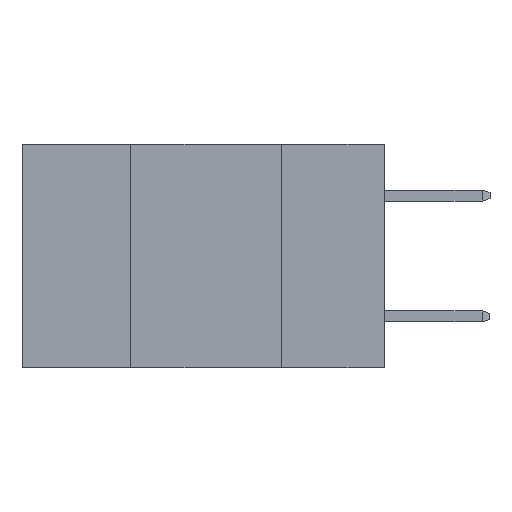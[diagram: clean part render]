
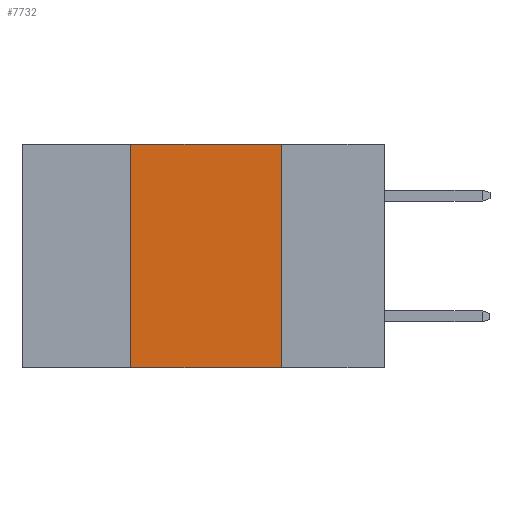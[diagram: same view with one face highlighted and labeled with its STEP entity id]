
A CAD part, left-side view. The second image highlights one B-rep face of the part: STEP entity #7732.
In plain terms, the highlighted planar face has unit normal (-1, 0, 0).
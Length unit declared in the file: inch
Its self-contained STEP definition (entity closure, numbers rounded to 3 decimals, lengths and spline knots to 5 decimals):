
#325 = EDGE_LOOP ( 'NONE', ( #2328, #1621, #1782, #8304 ) ) ;
#580 = DIRECTION ( 'NONE',  ( 0., -1., 0. ) ) ;
#707 = VERTEX_POINT ( 'NONE', #9486 ) ;
#1621 = ORIENTED_EDGE ( 'NONE', *, *, #9307, .F. ) ;
#1782 = ORIENTED_EDGE ( 'NONE', *, *, #3301, .F. ) ;
#2328 = ORIENTED_EDGE ( 'NONE', *, *, #10370, .F. ) ;
#2330 = DIRECTION ( 'NONE',  ( 0., -1., 0. ) ) ;
#2654 = LINE ( 'NONE', #12769, #10809 ) ;
#2722 = VERTEX_POINT ( 'NONE', #6945 ) ;
#3301 = EDGE_CURVE ( 'NONE', #11123, #3379, #5856, .T. ) ;
#3379 = VERTEX_POINT ( 'NONE', #12836 ) ;
#4495 = PLANE ( 'NONE',  #11572 ) ;
#4500 = CARTESIAN_POINT ( 'NONE',  ( 0., 0.42, -0.37 ) ) ;
#4861 = VECTOR ( 'NONE', #6802, 39.37008 ) ;
#5563 = DIRECTION ( 'NONE',  ( 1., 0., 0. ) ) ;
#5856 = LINE ( 'NONE', #11742, #4861 ) ;
#6130 = VECTOR ( 'NONE', #580, 39.37008 ) ;
#6672 = FACE_OUTER_BOUND ( 'NONE', #325, .T. ) ;
#6775 = VECTOR ( 'NONE', #2330, 39.37008 ) ;
#6802 = DIRECTION ( 'NONE',  ( 0., 0., 1. ) ) ;
#6945 = CARTESIAN_POINT ( 'NONE',  ( 0., 0.17, 0. ) ) ;
#7732 = ADVANCED_FACE ( 'NONE', ( #6672 ), #4495, .F. ) ;
#8263 = LINE ( 'NONE', #13473, #6130 ) ;
#8304 = ORIENTED_EDGE ( 'NONE', *, *, #13366, .T. ) ;
#9307 = EDGE_CURVE ( 'NONE', #3379, #2722, #8263, .T. ) ;
#9486 = CARTESIAN_POINT ( 'NONE',  ( 0., 0.17, -0.37 ) ) ;
#10370 = EDGE_CURVE ( 'NONE', #2722, #707, #2654, .T. ) ;
#10808 = CARTESIAN_POINT ( 'NONE',  ( 0., 0.6, -0.37 ) ) ;
#10809 = VECTOR ( 'NONE', #13818, 39.37008 ) ;
#11123 = VERTEX_POINT ( 'NONE', #4500 ) ;
#11572 = AXIS2_PLACEMENT_3D ( 'NONE', #11837, #5563, #12882 ) ;
#11742 = CARTESIAN_POINT ( 'NONE',  ( 0., 0.42, 0. ) ) ;
#11837 = CARTESIAN_POINT ( 'NONE',  ( 0., 0.6, 0. ) ) ;
#12006 = LINE ( 'NONE', #10808, #6775 ) ;
#12769 = CARTESIAN_POINT ( 'NONE',  ( 0., 0.17, 0. ) ) ;
#12836 = CARTESIAN_POINT ( 'NONE',  ( 0., 0.42, 0. ) ) ;
#12882 = DIRECTION ( 'NONE',  ( 0., 0., -1. ) ) ;
#13366 = EDGE_CURVE ( 'NONE', #11123, #707, #12006, .T. ) ;
#13473 = CARTESIAN_POINT ( 'NONE',  ( 0., 0.6, 0. ) ) ;
#13818 = DIRECTION ( 'NONE',  ( 0., 0., -1. ) ) ;
